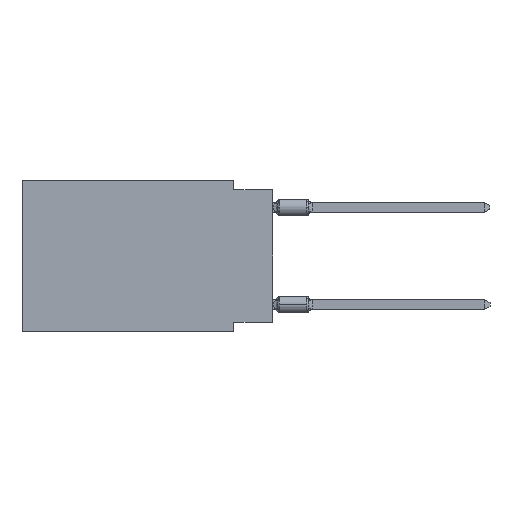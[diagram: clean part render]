
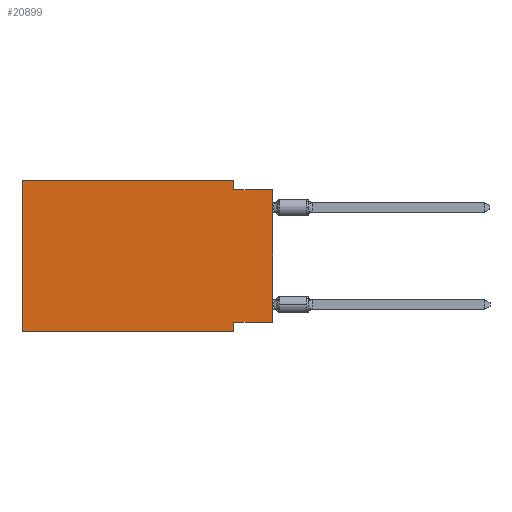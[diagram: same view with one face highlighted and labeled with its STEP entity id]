
A CAD part, left-side view. The second image highlights one B-rep face of the part: STEP entity #20899.
In plain terms, the highlighted planar face has unit normal (-1, 0, 0).
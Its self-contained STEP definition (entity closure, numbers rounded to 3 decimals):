
#278 = LINE ( 'NONE', #8616, #21213 ) ;
#570 = CARTESIAN_POINT ( 'NONE',  ( 0., 16.383, -9.906 ) ) ;
#967 = CARTESIAN_POINT ( 'NONE',  ( 0., 2.54, -9.906 ) ) ;
#1109 = VERTEX_POINT ( 'NONE', #13974 ) ;
#1356 = DIRECTION ( 'NONE',  ( 0., 1., 0. ) ) ;
#1375 = VERTEX_POINT ( 'NONE', #9158 ) ;
#1503 = EDGE_CURVE ( 'NONE', #1566, #1109, #4071, .T. ) ;
#1566 = VERTEX_POINT ( 'NONE', #11875 ) ;
#2704 = EDGE_LOOP ( 'NONE', ( #16514, #8327, #18592, #25867, #8193, #4888, #6853, #17437 ) ) ;
#2711 = LINE ( 'NONE', #15111, #11814 ) ;
#3686 = DIRECTION ( 'NONE',  ( 0., 0., -1. ) ) ;
#4071 = LINE ( 'NONE', #26840, #15596 ) ;
#4170 = CARTESIAN_POINT ( 'NONE',  ( 0., 2.54, -9.906 ) ) ;
#4653 = AXIS2_PLACEMENT_3D ( 'NONE', #26336, #16363, #3686 ) ;
#4888 = ORIENTED_EDGE ( 'NONE', *, *, #6047, .T. ) ;
#5518 = EDGE_CURVE ( 'NONE', #6639, #1375, #23130, .T. ) ;
#6047 = EDGE_CURVE ( 'NONE', #21208, #25327, #19274, .T. ) ;
#6286 = DIRECTION ( 'NONE',  ( 0., 0., -1. ) ) ;
#6393 = VECTOR ( 'NONE', #25553, 1000. ) ;
#6611 = VERTEX_POINT ( 'NONE', #9902 ) ;
#6639 = VERTEX_POINT ( 'NONE', #24238 ) ;
#6853 = ORIENTED_EDGE ( 'NONE', *, *, #24345, .F. ) ;
#7165 = VECTOR ( 'NONE', #6286, 1000. ) ;
#7794 = EDGE_CURVE ( 'NONE', #1566, #6611, #23627, .T. ) ;
#7931 = LINE ( 'NONE', #967, #7165 ) ;
#8050 = PLANE ( 'NONE',  #4653 ) ;
#8193 = ORIENTED_EDGE ( 'NONE', *, *, #15410, .F. ) ;
#8327 = ORIENTED_EDGE ( 'NONE', *, *, #25707, .F. ) ;
#8616 = CARTESIAN_POINT ( 'NONE',  ( 0., 2.54, 0. ) ) ;
#8766 = DIRECTION ( 'NONE',  ( 0., 0., -1. ) ) ;
#9158 = CARTESIAN_POINT ( 'NONE',  ( 0., 2.54, 0. ) ) ;
#9902 = CARTESIAN_POINT ( 'NONE',  ( 0., 0., -0.635 ) ) ;
#10134 = CARTESIAN_POINT ( 'NONE',  ( 0., 2.54, -0.635 ) ) ;
#11674 = CARTESIAN_POINT ( 'NONE',  ( 0., 0., -0.635 ) ) ;
#11814 = VECTOR ( 'NONE', #17162, 1000. ) ;
#11875 = CARTESIAN_POINT ( 'NONE',  ( 0., 0., -9.271 ) ) ;
#12151 = FACE_OUTER_BOUND ( 'NONE', #2704, .T. ) ;
#13974 = CARTESIAN_POINT ( 'NONE',  ( 0., 2.54, -9.271 ) ) ;
#14529 = DIRECTION ( 'NONE',  ( 0., -1., 0. ) ) ;
#15111 = CARTESIAN_POINT ( 'NONE',  ( 0., 16.383, 0. ) ) ;
#15410 = EDGE_CURVE ( 'NONE', #21208, #6639, #2711, .T. ) ;
#15596 = VECTOR ( 'NONE', #1356, 1000. ) ;
#16280 = LINE ( 'NONE', #11674, #21136 ) ;
#16363 = DIRECTION ( 'NONE',  ( 1., 0., 0. ) ) ;
#16514 = ORIENTED_EDGE ( 'NONE', *, *, #7794, .T. ) ;
#17162 = DIRECTION ( 'NONE',  ( 0., 0., 1. ) ) ;
#17340 = CARTESIAN_POINT ( 'NONE',  ( 0., 0., 0. ) ) ;
#17437 = ORIENTED_EDGE ( 'NONE', *, *, #1503, .F. ) ;
#18592 = ORIENTED_EDGE ( 'NONE', *, *, #20699, .F. ) ;
#19171 = VECTOR ( 'NONE', #21722, 1000. ) ;
#19274 = LINE ( 'NONE', #570, #6393 ) ;
#19370 = CARTESIAN_POINT ( 'NONE',  ( 0., 16.383, -9.906 ) ) ;
#19872 = VECTOR ( 'NONE', #14529, 1000. ) ;
#20473 = VERTEX_POINT ( 'NONE', #10134 ) ;
#20699 = EDGE_CURVE ( 'NONE', #1375, #20473, #278, .T. ) ;
#20899 = ADVANCED_FACE ( 'NONE', ( #12151 ), #8050, .F. ) ;
#21136 = VECTOR ( 'NONE', #24610, 1000. ) ;
#21208 = VERTEX_POINT ( 'NONE', #19370 ) ;
#21213 = VECTOR ( 'NONE', #8766, 1000. ) ;
#21722 = DIRECTION ( 'NONE',  ( 0., 0., 1. ) ) ;
#23130 = LINE ( 'NONE', #25312, #19872 ) ;
#23627 = LINE ( 'NONE', #17340, #19171 ) ;
#24238 = CARTESIAN_POINT ( 'NONE',  ( 0., 16.383, 0. ) ) ;
#24345 = EDGE_CURVE ( 'NONE', #1109, #25327, #7931, .T. ) ;
#24610 = DIRECTION ( 'NONE',  ( 0., -1., 0. ) ) ;
#25312 = CARTESIAN_POINT ( 'NONE',  ( 0., 16.383, 0. ) ) ;
#25327 = VERTEX_POINT ( 'NONE', #4170 ) ;
#25553 = DIRECTION ( 'NONE',  ( 0., -1., 0. ) ) ;
#25707 = EDGE_CURVE ( 'NONE', #20473, #6611, #16280, .T. ) ;
#25867 = ORIENTED_EDGE ( 'NONE', *, *, #5518, .F. ) ;
#26336 = CARTESIAN_POINT ( 'NONE',  ( 0., 16.383, 0. ) ) ;
#26840 = CARTESIAN_POINT ( 'NONE',  ( 0., 0., -9.271 ) ) ;
